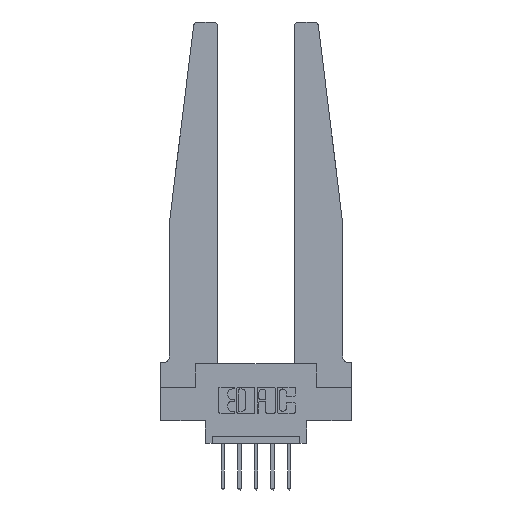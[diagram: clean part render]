
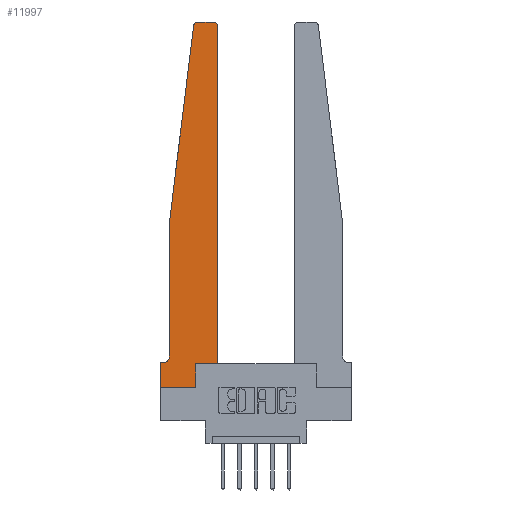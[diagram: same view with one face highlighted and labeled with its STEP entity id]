
A CAD part, top view. The second image highlights one B-rep face of the part: STEP entity #11997.
In plain terms, the highlighted planar face has unit normal (0, 0, 1).
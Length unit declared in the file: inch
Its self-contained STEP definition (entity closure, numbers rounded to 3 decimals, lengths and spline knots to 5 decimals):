
#8 = ORIENTED_EDGE ( 'NONE', *, *, #5917, .T. ) ;
#20 = ORIENTED_EDGE ( 'NONE', *, *, #6140, .T. ) ;
#250 = CARTESIAN_POINT ( 'NONE',  ( 0., 0.1875, 0.37 ) ) ;
#417 = DIRECTION ( 'NONE',  ( -1., 0., 0. ) ) ;
#775 = VERTEX_POINT ( 'NONE', #8872 ) ;
#895 = DIRECTION ( 'NONE',  ( 1., 0., 0. ) ) ;
#1019 = VERTEX_POINT ( 'NONE', #3267 ) ;
#1024 = VECTOR ( 'NONE', #4853, 39.37008 ) ;
#1048 = VERTEX_POINT ( 'NONE', #1659 ) ;
#1051 = CARTESIAN_POINT ( 'NONE',  ( 0.015, 0.1875, 0.37 ) ) ;
#1124 = CARTESIAN_POINT ( 'NONE',  ( 0.25, 2.75, 0.37 ) ) ;
#1619 = CARTESIAN_POINT ( 'NONE',  ( 0.2605, 0.18, 0.37 ) ) ;
#1659 = CARTESIAN_POINT ( 'NONE',  ( 0.425, 2.72, 0.37 ) ) ;
#1671 = CIRCLE ( 'NONE', #7777, 0.03 ) ;
#1749 = DIRECTION ( 'NONE',  ( -0.122, -0.992, 0. ) ) ;
#1905 = AXIS2_PLACEMENT_3D ( 'NONE', #6708, #8531, #417 ) ;
#2244 = LINE ( 'NONE', #10406, #4732 ) ;
#2256 = LINE ( 'NONE', #3210, #2337 ) ;
#2330 = VERTEX_POINT ( 'NONE', #12245 ) ;
#2337 = VECTOR ( 'NONE', #7395, 39.37008 ) ;
#2366 = AXIS2_PLACEMENT_3D ( 'NONE', #250, #5519, #4251 ) ;
#2442 = EDGE_LOOP ( 'NONE', ( #9994, #12460, #7624, #9251, #10715, #3352, #7388, #8, #6656, #2477, #6361, #20 ) ) ;
#2473 = DIRECTION ( 'NONE',  ( 1., 0., 0. ) ) ;
#2477 = ORIENTED_EDGE ( 'NONE', *, *, #9687, .T. ) ;
#2796 = CARTESIAN_POINT ( 'NONE',  ( 0.24675, 2.72367, 0.37 ) ) ;
#2843 = FACE_OUTER_BOUND ( 'NONE', #2442, .T. ) ;
#3084 = EDGE_CURVE ( 'NONE', #5248, #4725, #2244, .T. ) ;
#3163 = DIRECTION ( 'NONE',  ( -1., 0., 0. ) ) ;
#3210 = CARTESIAN_POINT ( 'NONE',  ( 0., 0., 0.37 ) ) ;
#3267 = CARTESIAN_POINT ( 'NONE',  ( 0.27653, 2.75, 0.37 ) ) ;
#3291 = CARTESIAN_POINT ( 'NONE',  ( 0.27653, 2.72, 0.37 ) ) ;
#3352 = ORIENTED_EDGE ( 'NONE', *, *, #6542, .T. ) ;
#3693 = DIRECTION ( 'NONE',  ( 0., 1., 0. ) ) ;
#3890 = VECTOR ( 'NONE', #3163, 39.37008 ) ;
#4041 = EDGE_CURVE ( 'NONE', #4859, #9658, #9681, .T. ) ;
#4132 = CARTESIAN_POINT ( 'NONE',  ( 0., 0., 0.37 ) ) ;
#4246 = DIRECTION ( 'NONE',  ( 0., 1., 0. ) ) ;
#4251 = DIRECTION ( 'NONE',  ( 1., 0., 0. ) ) ;
#4725 = VERTEX_POINT ( 'NONE', #9084 ) ;
#4732 = VECTOR ( 'NONE', #6369, 39.37008 ) ;
#4752 = LINE ( 'NONE', #10855, #6854 ) ;
#4828 = CARTESIAN_POINT ( 'NONE',  ( 0., 0., 0.37 ) ) ;
#4853 = DIRECTION ( 'NONE',  ( -1., 0., 0. ) ) ;
#4859 = VERTEX_POINT ( 'NONE', #7520 ) ;
#5248 = VERTEX_POINT ( 'NONE', #6297 ) ;
#5519 = DIRECTION ( 'NONE',  ( 0., 0., 1. ) ) ;
#5821 = LINE ( 'NONE', #8907, #1024 ) ;
#5841 = VERTEX_POINT ( 'NONE', #8477 ) ;
#5917 = EDGE_CURVE ( 'NONE', #9658, #5841, #2256, .T. ) ;
#6139 = DIRECTION ( 'NONE',  ( 0., 0., 1. ) ) ;
#6140 = EDGE_CURVE ( 'NONE', #1048, #6899, #1671, .T. ) ;
#6297 = CARTESIAN_POINT ( 'NONE',  ( 0.065, 1.25, 0.37 ) ) ;
#6361 = ORIENTED_EDGE ( 'NONE', *, *, #12086, .T. ) ;
#6369 = DIRECTION ( 'NONE',  ( 0., -1., 0. ) ) ;
#6419 = AXIS2_PLACEMENT_3D ( 'NONE', #3291, #6139, #895 ) ;
#6435 = DIRECTION ( 'NONE',  ( 0., 0., 1. ) ) ;
#6501 = DIRECTION ( 'NONE',  ( 1., 0., 0. ) ) ;
#6542 = EDGE_CURVE ( 'NONE', #12394, #4859, #5821, .T. ) ;
#6545 = VECTOR ( 'NONE', #1749, 39.37008 ) ;
#6656 = ORIENTED_EDGE ( 'NONE', *, *, #10962, .T. ) ;
#6708 = CARTESIAN_POINT ( 'NONE',  ( 0.015, 0.2375, 0.37 ) ) ;
#6781 = LINE ( 'NONE', #1619, #10589 ) ;
#6854 = VECTOR ( 'NONE', #2473, 39.37008 ) ;
#6899 = VERTEX_POINT ( 'NONE', #13109 ) ;
#7018 = PLANE ( 'NONE',  #2366 ) ;
#7334 = EDGE_CURVE ( 'NONE', #4725, #12394, #10846, .T. ) ;
#7388 = ORIENTED_EDGE ( 'NONE', *, *, #4041, .T. ) ;
#7395 = DIRECTION ( 'NONE',  ( 1., 0., 0. ) ) ;
#7520 = CARTESIAN_POINT ( 'NONE',  ( 0., 0.1875, 0.37 ) ) ;
#7624 = ORIENTED_EDGE ( 'NONE', *, *, #11389, .T. ) ;
#7777 = AXIS2_PLACEMENT_3D ( 'NONE', #10459, #6435, #6501 ) ;
#8301 = DIRECTION ( 'NONE',  ( 0., -1., 0. ) ) ;
#8308 = LINE ( 'NONE', #1124, #3890 ) ;
#8477 = CARTESIAN_POINT ( 'NONE',  ( 0.2605, 0., 0.37 ) ) ;
#8531 = DIRECTION ( 'NONE',  ( 0., 0., -1. ) ) ;
#8872 = CARTESIAN_POINT ( 'NONE',  ( 0.2605, 0.18, 0.37 ) ) ;
#8907 = CARTESIAN_POINT ( 'NONE',  ( 0.065, 0.1875, 0.37 ) ) ;
#9084 = CARTESIAN_POINT ( 'NONE',  ( 0.065, 0.2375, 0.37 ) ) ;
#9173 = LINE ( 'NONE', #12415, #6545 ) ;
#9251 = ORIENTED_EDGE ( 'NONE', *, *, #3084, .T. ) ;
#9658 = VERTEX_POINT ( 'NONE', #4828 ) ;
#9681 = LINE ( 'NONE', #4132, #10806 ) ;
#9687 = EDGE_CURVE ( 'NONE', #775, #2330, #4752, .T. ) ;
#9994 = ORIENTED_EDGE ( 'NONE', *, *, #12346, .T. ) ;
#10406 = CARTESIAN_POINT ( 'NONE',  ( 0.065, 1.25, 0.37 ) ) ;
#10459 = CARTESIAN_POINT ( 'NONE',  ( 0.395, 2.72, 0.37 ) ) ;
#10589 = VECTOR ( 'NONE', #3693, 39.37008 ) ;
#10715 = ORIENTED_EDGE ( 'NONE', *, *, #7334, .T. ) ;
#10806 = VECTOR ( 'NONE', #8301, 39.37008 ) ;
#10846 = CIRCLE ( 'NONE', #1905, 0.05 ) ;
#10855 = CARTESIAN_POINT ( 'NONE',  ( 0.425, 0.18, 0.37 ) ) ;
#10962 = EDGE_CURVE ( 'NONE', #5841, #775, #6781, .T. ) ;
#10979 = VERTEX_POINT ( 'NONE', #2796 ) ;
#11389 = EDGE_CURVE ( 'NONE', #10979, #5248, #9173, .T. ) ;
#11997 = ADVANCED_FACE ( 'NONE', ( #2843 ), #7018, .T. ) ;
#12086 = EDGE_CURVE ( 'NONE', #2330, #1048, #12500, .T. ) ;
#12245 = CARTESIAN_POINT ( 'NONE',  ( 0.425, 0.18, 0.37 ) ) ;
#12262 = CIRCLE ( 'NONE', #6419, 0.03 ) ;
#12346 = EDGE_CURVE ( 'NONE', #6899, #1019, #8308, .T. ) ;
#12394 = VERTEX_POINT ( 'NONE', #1051 ) ;
#12415 = CARTESIAN_POINT ( 'NONE',  ( 0.065, 1.25, 0.37 ) ) ;
#12460 = ORIENTED_EDGE ( 'NONE', *, *, #13117, .T. ) ;
#12500 = LINE ( 'NONE', #13440, #12802 ) ;
#12802 = VECTOR ( 'NONE', #4246, 39.37008 ) ;
#13109 = CARTESIAN_POINT ( 'NONE',  ( 0.395, 2.75, 0.37 ) ) ;
#13117 = EDGE_CURVE ( 'NONE', #1019, #10979, #12262, .T. ) ;
#13440 = CARTESIAN_POINT ( 'NONE',  ( 0.425, 0.18, 0.37 ) ) ;
